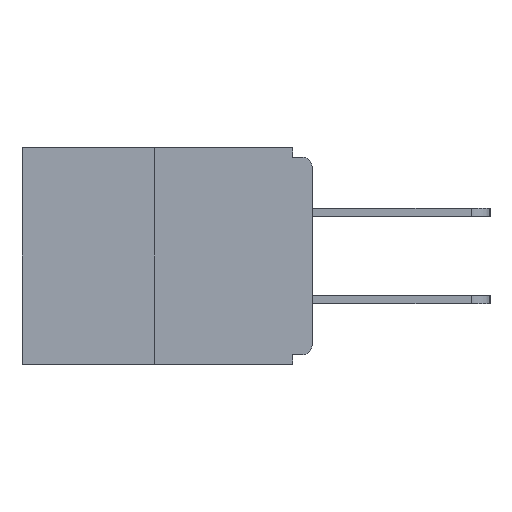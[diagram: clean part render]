
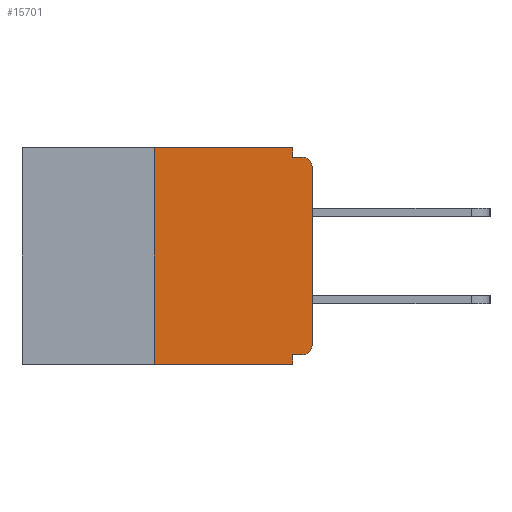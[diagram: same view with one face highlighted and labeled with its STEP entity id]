
A CAD part, left-side view. The second image highlights one B-rep face of the part: STEP entity #15701.
In plain terms, the highlighted planar face has unit normal (-1, 0, 0).
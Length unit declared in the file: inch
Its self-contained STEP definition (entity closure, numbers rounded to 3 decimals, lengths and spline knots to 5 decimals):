
#281 = DIRECTION ( 'NONE',  ( 0., 0., 1. ) ) ;
#377 = EDGE_CURVE ( 'NONE', #3227, #1357, #17609, .T. ) ;
#665 = VERTEX_POINT ( 'NONE', #6329 ) ;
#966 = LINE ( 'NONE', #10054, #13469 ) ;
#1045 = VECTOR ( 'NONE', #7963, 39.37008 ) ;
#1165 = EDGE_CURVE ( 'NONE', #665, #13981, #16532, .T. ) ;
#1233 = LINE ( 'NONE', #11736, #6928 ) ;
#1357 = VERTEX_POINT ( 'NONE', #2244 ) ;
#2244 = CARTESIAN_POINT ( 'NONE',  ( 0., 0.031, -0.015 ) ) ;
#2256 = DIRECTION ( 'NONE',  ( -1., 0., 0. ) ) ;
#2258 = VERTEX_POINT ( 'NONE', #12512 ) ;
#2816 = ORIENTED_EDGE ( 'NONE', *, *, #16053, .F. ) ;
#2818 = DIRECTION ( 'NONE',  ( 0., 0., -1. ) ) ;
#2918 = CARTESIAN_POINT ( 'NONE',  ( 0., 0.031, -0.343 ) ) ;
#3017 = ORIENTED_EDGE ( 'NONE', *, *, #5932, .F. ) ;
#3227 = VERTEX_POINT ( 'NONE', #10243 ) ;
#3453 = DIRECTION ( 'NONE',  ( 0., -1., 0. ) ) ;
#3851 = LINE ( 'NONE', #7889, #7245 ) ;
#4025 = CARTESIAN_POINT ( 'NONE',  ( 0., 0.015, -0.313 ) ) ;
#4032 = DIRECTION ( 'NONE',  ( 1., 0., 0. ) ) ;
#4417 = DIRECTION ( 'NONE',  ( 0., 0., 1. ) ) ;
#4707 = ORIENTED_EDGE ( 'NONE', *, *, #1165, .T. ) ;
#4798 = VECTOR ( 'NONE', #5203, 39.37008 ) ;
#5043 = CARTESIAN_POINT ( 'NONE',  ( 0., 0., -0.328 ) ) ;
#5203 = DIRECTION ( 'NONE',  ( 0., -1., 0. ) ) ;
#5329 = LINE ( 'NONE', #5043, #12148 ) ;
#5602 = CARTESIAN_POINT ( 'NONE',  ( 0., 0.015, -0.015 ) ) ;
#5822 = CIRCLE ( 'NONE', #7951, 0.015 ) ;
#5932 = EDGE_CURVE ( 'NONE', #2258, #3227, #16524, .T. ) ;
#6093 = VERTEX_POINT ( 'NONE', #11733 ) ;
#6329 = CARTESIAN_POINT ( 'NONE',  ( 0., 0.015, -0.328 ) ) ;
#6682 = EDGE_CURVE ( 'NONE', #18727, #9885, #5822, .T. ) ;
#6807 = ORIENTED_EDGE ( 'NONE', *, *, #16231, .F. ) ;
#6928 = VECTOR ( 'NONE', #281, 39.37008 ) ;
#7245 = VECTOR ( 'NONE', #3453, 39.37008 ) ;
#7375 = ORIENTED_EDGE ( 'NONE', *, *, #10424, .T. ) ;
#7889 = CARTESIAN_POINT ( 'NONE',  ( 0., 0.46, -0.343 ) ) ;
#7951 = AXIS2_PLACEMENT_3D ( 'NONE', #18211, #2256, #10893 ) ;
#7963 = DIRECTION ( 'NONE',  ( 0., -1., 0. ) ) ;
#7999 = CARTESIAN_POINT ( 'NONE',  ( 0., 0.031, -0.343 ) ) ;
#8049 = EDGE_CURVE ( 'NONE', #6093, #8883, #3851, .T. ) ;
#8364 = DIRECTION ( 'NONE',  ( 0., 0., -1. ) ) ;
#8486 = PLANE ( 'NONE',  #17526 ) ;
#8683 = LINE ( 'NONE', #12379, #4798 ) ;
#8883 = VERTEX_POINT ( 'NONE', #7999 ) ;
#9885 = VERTEX_POINT ( 'NONE', #5602 ) ;
#9989 = CARTESIAN_POINT ( 'NONE',  ( 0., 0.031, -0.328 ) ) ;
#10054 = CARTESIAN_POINT ( 'NONE',  ( 0., 0., 0. ) ) ;
#10243 = CARTESIAN_POINT ( 'NONE',  ( 0., 0.031, 0. ) ) ;
#10424 = EDGE_CURVE ( 'NONE', #13981, #18727, #966, .T. ) ;
#10893 = DIRECTION ( 'NONE',  ( 0., 0., -1. ) ) ;
#10919 = ORIENTED_EDGE ( 'NONE', *, *, #17686, .F. ) ;
#11073 = EDGE_LOOP ( 'NONE', ( #3017, #2816, #14797, #16177, #6807, #4707, #7375, #12808, #10919, #13371 ) ) ;
#11499 = LINE ( 'NONE', #2918, #11711 ) ;
#11711 = VECTOR ( 'NONE', #17389, 39.37008 ) ;
#11733 = CARTESIAN_POINT ( 'NONE',  ( 0., 0.25, -0.343 ) ) ;
#11736 = CARTESIAN_POINT ( 'NONE',  ( 0., 0.25, 0. ) ) ;
#12148 = VECTOR ( 'NONE', #15230, 39.37008 ) ;
#12379 = CARTESIAN_POINT ( 'NONE',  ( 0., 0., -0.015 ) ) ;
#12512 = CARTESIAN_POINT ( 'NONE',  ( 0., 0.25, 0. ) ) ;
#12808 = ORIENTED_EDGE ( 'NONE', *, *, #6682, .T. ) ;
#13371 = ORIENTED_EDGE ( 'NONE', *, *, #377, .F. ) ;
#13469 = VECTOR ( 'NONE', #4417, 39.37008 ) ;
#13981 = VERTEX_POINT ( 'NONE', #15354 ) ;
#14086 = CARTESIAN_POINT ( 'NONE',  ( 0., 0.46, 0. ) ) ;
#14200 = DIRECTION ( 'NONE',  ( -1., 0., 0. ) ) ;
#14467 = CARTESIAN_POINT ( 'NONE',  ( 0., 0.031, 0. ) ) ;
#14797 = ORIENTED_EDGE ( 'NONE', *, *, #8049, .T. ) ;
#15103 = EDGE_CURVE ( 'NONE', #17481, #8883, #11499, .T. ) ;
#15127 = FACE_OUTER_BOUND ( 'NONE', #11073, .T. ) ;
#15230 = DIRECTION ( 'NONE',  ( 0., 1., 0. ) ) ;
#15295 = AXIS2_PLACEMENT_3D ( 'NONE', #4025, #14200, #2818 ) ;
#15354 = CARTESIAN_POINT ( 'NONE',  ( 0., 0., -0.313 ) ) ;
#15483 = DIRECTION ( 'NONE',  ( 0., 0., -1. ) ) ;
#15701 = ADVANCED_FACE ( 'NONE', ( #15127 ), #8486, .F. ) ;
#16053 = EDGE_CURVE ( 'NONE', #6093, #2258, #1233, .T. ) ;
#16177 = ORIENTED_EDGE ( 'NONE', *, *, #15103, .F. ) ;
#16231 = EDGE_CURVE ( 'NONE', #665, #17481, #5329, .T. ) ;
#16417 = CARTESIAN_POINT ( 'NONE',  ( 0., 0.46, 0. ) ) ;
#16524 = LINE ( 'NONE', #16417, #1045 ) ;
#16532 = CIRCLE ( 'NONE', #15295, 0.015 ) ;
#17389 = DIRECTION ( 'NONE',  ( 0., 0., -1. ) ) ;
#17402 = VECTOR ( 'NONE', #15483, 39.37008 ) ;
#17481 = VERTEX_POINT ( 'NONE', #9989 ) ;
#17526 = AXIS2_PLACEMENT_3D ( 'NONE', #14086, #4032, #8364 ) ;
#17609 = LINE ( 'NONE', #14467, #17402 ) ;
#17686 = EDGE_CURVE ( 'NONE', #1357, #9885, #8683, .T. ) ;
#18211 = CARTESIAN_POINT ( 'NONE',  ( 0., 0.015, -0.03 ) ) ;
#18347 = CARTESIAN_POINT ( 'NONE',  ( 0., 0., -0.03 ) ) ;
#18727 = VERTEX_POINT ( 'NONE', #18347 ) ;
